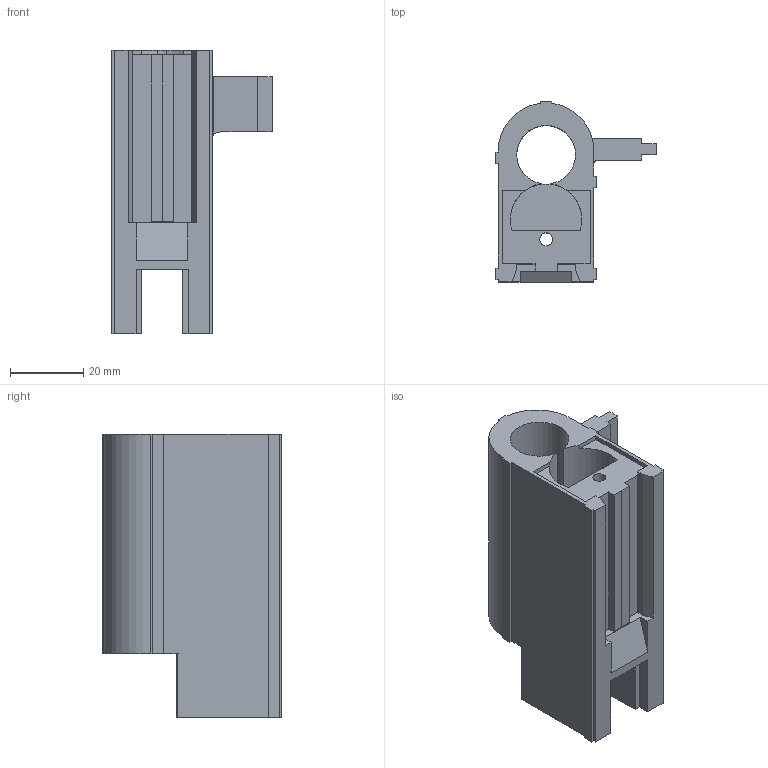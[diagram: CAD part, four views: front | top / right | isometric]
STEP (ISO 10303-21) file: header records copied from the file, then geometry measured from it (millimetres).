
FILE_DESCRIPTION(('FreeCAD Model'),'2;1');
FILE_NAME('Open CASCADE Shape Model','2021-04-08T19:56:35',('Author'),( ''),'Open CASCADE STEP processor 7.5','FreeCAD','Unknown');
FILE_SCHEMA(('AUTOMOTIVE_DESIGN { 1 0 10303 214 1 1 1 1 }'));
Length unit declared in the file: millimetre
Products named in the file (1): Fillet001
Bounding box: 43.7 x 49.01 x 77.25 mm (x, y, z)
Volume: 52382.3 mm3; surface area: 20794.4 mm2
Topology: 1 solids, 1 shells, 95 faces, 277 edges, 185 vertices
Faces by surface type: plane 81, cylinder 13, torus 1
Full cylindrical faces by diameter (mm): 3 x1, 3.5 x1, 5 x2, 6.5 x1, 16 x1
Entity records: 7420 total; most frequent: CARTESIAN_POINT 2047, DIRECTION 932, LINE 658, VECTOR 658, ORIENTED_EDGE 554, PCURVE 554, DEFINITIONAL_REPRESENTATION 554, EDGE_CURVE 277
